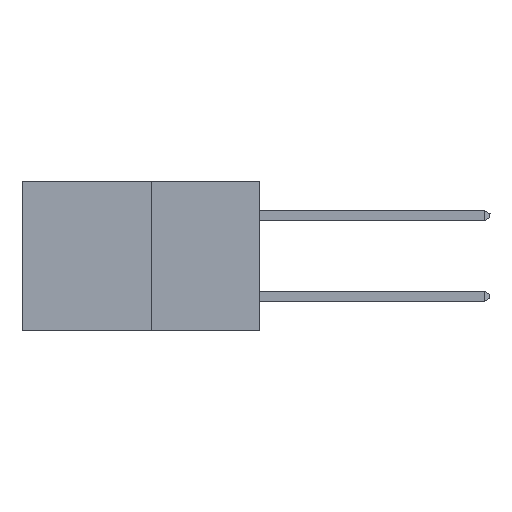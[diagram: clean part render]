
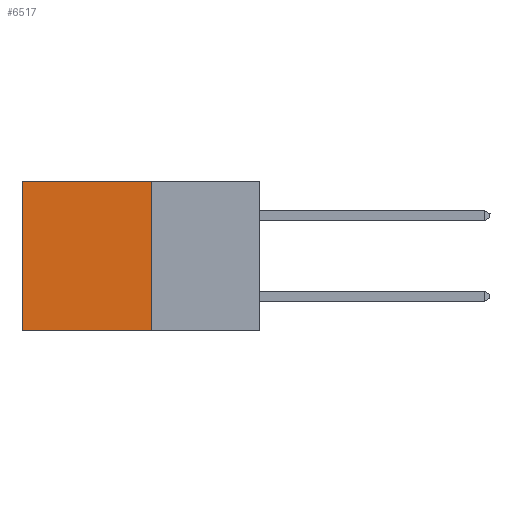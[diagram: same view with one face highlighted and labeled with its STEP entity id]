
A CAD part, left-side view. The second image highlights one B-rep face of the part: STEP entity #6517.
In plain terms, the highlighted planar face has unit normal (-1, 0, 0).
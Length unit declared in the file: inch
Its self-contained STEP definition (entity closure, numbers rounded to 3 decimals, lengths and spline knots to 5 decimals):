
#1467 = CARTESIAN_POINT ( 'NONE',  ( 0.277, 0.27, -0.37 ) ) ;
#1622 = CARTESIAN_POINT ( 'NONE',  ( 0.277, 0.27, -0.37 ) ) ;
#1843 = LINE ( 'NONE', #1622, #6946 ) ;
#2416 = LINE ( 'NONE', #8705, #9237 ) ;
#2488 = VECTOR ( 'NONE', #6010, 39.37008 ) ;
#3140 = VERTEX_POINT ( 'NONE', #8207 ) ;
#3151 = EDGE_CURVE ( 'NONE', #10975, #7313, #1843, .T. ) ;
#3200 = CARTESIAN_POINT ( 'NONE',  ( 0.277, 0.27, 0. ) ) ;
#3613 = DIRECTION ( 'NONE',  ( 0., 0., -1. ) ) ;
#3728 = EDGE_CURVE ( 'NONE', #7313, #11199, #2416, .T. ) ;
#3983 = VECTOR ( 'NONE', #10937, 39.37008 ) ;
#4176 = ORIENTED_EDGE ( 'NONE', *, *, #7122, .T. ) ;
#4209 = ORIENTED_EDGE ( 'NONE', *, *, #8098, .T. ) ;
#4281 = LINE ( 'NONE', #7677, #3983 ) ;
#6010 = DIRECTION ( 'NONE',  ( 0., 1., 0. ) ) ;
#6517 = ADVANCED_FACE ( 'NONE', ( #7858 ), #9924, .F. ) ;
#6946 = VECTOR ( 'NONE', #10243, 39.37008 ) ;
#7122 = EDGE_CURVE ( 'NONE', #3140, #11199, #4281, .T. ) ;
#7313 = VERTEX_POINT ( 'NONE', #1467 ) ;
#7470 = CARTESIAN_POINT ( 'NONE',  ( 0.277, 0.27, -0.37 ) ) ;
#7677 = CARTESIAN_POINT ( 'NONE',  ( 0.277, 0.59, -0.37 ) ) ;
#7858 = FACE_OUTER_BOUND ( 'NONE', #10090, .T. ) ;
#7960 = LINE ( 'NONE', #10395, #2488 ) ;
#8098 = EDGE_CURVE ( 'NONE', #10975, #3140, #7960, .T. ) ;
#8174 = CARTESIAN_POINT ( 'NONE',  ( 0.277, 0.59, -0.37 ) ) ;
#8207 = CARTESIAN_POINT ( 'NONE',  ( 0.277, 0.59, 0. ) ) ;
#8705 = CARTESIAN_POINT ( 'NONE',  ( 0.277, 0.27, -0.37 ) ) ;
#8706 = ORIENTED_EDGE ( 'NONE', *, *, #3151, .F. ) ;
#9154 = DIRECTION ( 'NONE',  ( 1., 0., 0. ) ) ;
#9237 = VECTOR ( 'NONE', #9719, 39.37008 ) ;
#9719 = DIRECTION ( 'NONE',  ( 0., 1., 0. ) ) ;
#9924 = PLANE ( 'NONE',  #9998 ) ;
#9998 = AXIS2_PLACEMENT_3D ( 'NONE', #7470, #9154, #3613 ) ;
#10090 = EDGE_LOOP ( 'NONE', ( #4176, #11193, #8706, #4209 ) ) ;
#10243 = DIRECTION ( 'NONE',  ( 0., 0., -1. ) ) ;
#10395 = CARTESIAN_POINT ( 'NONE',  ( 0.277, 0.27, 0. ) ) ;
#10937 = DIRECTION ( 'NONE',  ( 0., 0., -1. ) ) ;
#10975 = VERTEX_POINT ( 'NONE', #3200 ) ;
#11193 = ORIENTED_EDGE ( 'NONE', *, *, #3728, .F. ) ;
#11199 = VERTEX_POINT ( 'NONE', #8174 ) ;
